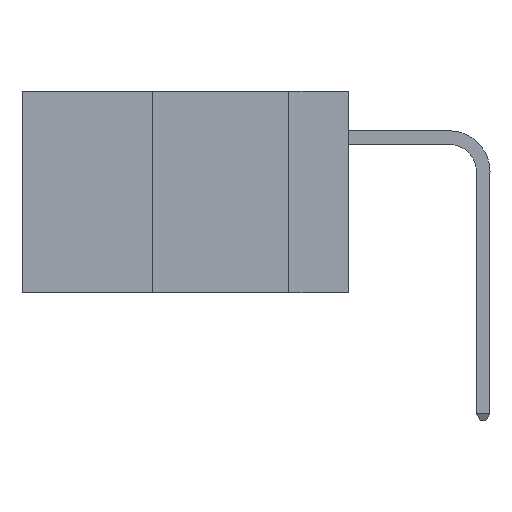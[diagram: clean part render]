
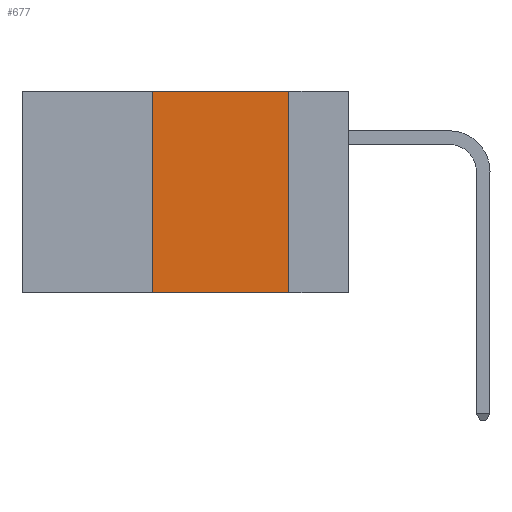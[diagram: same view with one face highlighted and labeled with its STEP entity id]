
A CAD part, left-side view. The second image highlights one B-rep face of the part: STEP entity #677.
In plain terms, the highlighted planar face has unit normal (-1, 0, 0).
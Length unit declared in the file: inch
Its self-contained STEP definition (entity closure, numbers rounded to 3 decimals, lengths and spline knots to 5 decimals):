
#311 = CARTESIAN_POINT ( 'NONE',  ( 0., 0.6, 0. ) ) ;
#677 = ADVANCED_FACE ( 'NONE', ( #11353 ), #1635, .F. ) ;
#901 = VECTOR ( 'NONE', #8963, 39.37008 ) ;
#1635 = PLANE ( 'NONE',  #11520 ) ;
#1887 = ORIENTED_EDGE ( 'NONE', *, *, #9330, .F. ) ;
#2023 = VECTOR ( 'NONE', #8884, 39.37008 ) ;
#2464 = CARTESIAN_POINT ( 'NONE',  ( 0., 0.11, 0. ) ) ;
#2574 = DIRECTION ( 'NONE',  ( 0., 0., 1. ) ) ;
#3277 = LINE ( 'NONE', #2464, #901 ) ;
#3517 = DIRECTION ( 'NONE',  ( 0., 0., -1. ) ) ;
#3632 = LINE ( 'NONE', #311, #2023 ) ;
#3669 = VECTOR ( 'NONE', #2574, 39.37008 ) ;
#3821 = CARTESIAN_POINT ( 'NONE',  ( 0., 0.11, -0.37 ) ) ;
#4157 = VERTEX_POINT ( 'NONE', #3821 ) ;
#4236 = DIRECTION ( 'NONE',  ( 0., -1., 0. ) ) ;
#4736 = CARTESIAN_POINT ( 'NONE',  ( 0., 0.36, -0.37 ) ) ;
#4762 = EDGE_CURVE ( 'NONE', #8642, #4157, #7943, .T. ) ;
#5043 = ORIENTED_EDGE ( 'NONE', *, *, #7189, .F. ) ;
#5554 = EDGE_CURVE ( 'NONE', #10545, #4157, #3277, .T. ) ;
#6595 = VERTEX_POINT ( 'NONE', #9635 ) ;
#6855 = LINE ( 'NONE', #8314, #3669 ) ;
#7189 = EDGE_CURVE ( 'NONE', #8642, #6595, #6855, .T. ) ;
#7204 = EDGE_LOOP ( 'NONE', ( #7711, #1887, #5043, #8266 ) ) ;
#7711 = ORIENTED_EDGE ( 'NONE', *, *, #5554, .F. ) ;
#7943 = LINE ( 'NONE', #8027, #11291 ) ;
#8027 = CARTESIAN_POINT ( 'NONE',  ( 0., 0.6, -0.37 ) ) ;
#8266 = ORIENTED_EDGE ( 'NONE', *, *, #4762, .T. ) ;
#8314 = CARTESIAN_POINT ( 'NONE',  ( 0., 0.36, 0. ) ) ;
#8642 = VERTEX_POINT ( 'NONE', #4736 ) ;
#8862 = CARTESIAN_POINT ( 'NONE',  ( 0., 0.11, 0. ) ) ;
#8884 = DIRECTION ( 'NONE',  ( 0., -1., 0. ) ) ;
#8963 = DIRECTION ( 'NONE',  ( 0., 0., -1. ) ) ;
#9330 = EDGE_CURVE ( 'NONE', #6595, #10545, #3632, .T. ) ;
#9635 = CARTESIAN_POINT ( 'NONE',  ( 0., 0.36, 0. ) ) ;
#10545 = VERTEX_POINT ( 'NONE', #8862 ) ;
#10854 = CARTESIAN_POINT ( 'NONE',  ( 0., 0.6, 0. ) ) ;
#11291 = VECTOR ( 'NONE', #4236, 39.37008 ) ;
#11353 = FACE_OUTER_BOUND ( 'NONE', #7204, .T. ) ;
#11520 = AXIS2_PLACEMENT_3D ( 'NONE', #10854, #11846, #3517 ) ;
#11846 = DIRECTION ( 'NONE',  ( 1., 0., 0. ) ) ;
